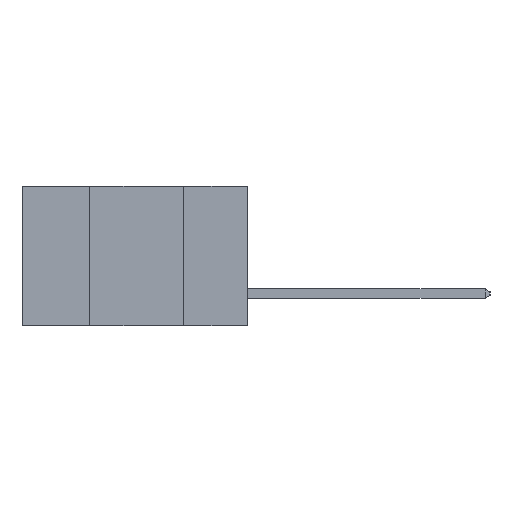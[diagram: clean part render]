
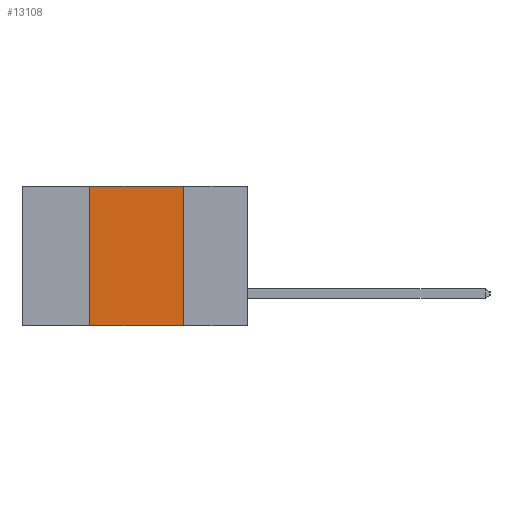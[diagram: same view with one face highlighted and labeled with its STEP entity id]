
A CAD part, left-side view. The second image highlights one B-rep face of the part: STEP entity #13108.
In plain terms, the highlighted planar face has unit normal (-1, 0, 0).
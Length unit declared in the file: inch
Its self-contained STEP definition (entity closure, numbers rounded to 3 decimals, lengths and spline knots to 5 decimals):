
#719 = EDGE_CURVE ( 'NONE', #11733, #8810, #9174, .T. ) ;
#1313 = VECTOR ( 'NONE', #2864, 39.37008 ) ;
#1465 = VECTOR ( 'NONE', #12414, 39.37008 ) ;
#2864 = DIRECTION ( 'NONE',  ( 0., 0., 1. ) ) ;
#2872 = CARTESIAN_POINT ( 'NONE',  ( 0., 0.42, -0.37 ) ) ;
#3395 = ORIENTED_EDGE ( 'NONE', *, *, #7102, .F. ) ;
#3495 = CARTESIAN_POINT ( 'NONE',  ( 0., 0.42, -0.37 ) ) ;
#3544 = ORIENTED_EDGE ( 'NONE', *, *, #719, .T. ) ;
#3562 = AXIS2_PLACEMENT_3D ( 'NONE', #10166, #4051, #11167 ) ;
#3681 = ORIENTED_EDGE ( 'NONE', *, *, #6445, .F. ) ;
#4051 = DIRECTION ( 'NONE',  ( 1., 0., 0. ) ) ;
#4271 = VERTEX_POINT ( 'NONE', #12427 ) ;
#5142 = LINE ( 'NONE', #10914, #7235 ) ;
#6215 = FACE_OUTER_BOUND ( 'NONE', #8141, .T. ) ;
#6445 = EDGE_CURVE ( 'NONE', #4271, #8810, #5142, .T. ) ;
#6952 = ORIENTED_EDGE ( 'NONE', *, *, #10053, .F. ) ;
#7055 = LINE ( 'NONE', #12461, #1465 ) ;
#7065 = CARTESIAN_POINT ( 'NONE',  ( 0., 0.42, 0. ) ) ;
#7102 = EDGE_CURVE ( 'NONE', #9390, #4271, #7055, .T. ) ;
#7235 = VECTOR ( 'NONE', #10649, 39.37008 ) ;
#8141 = EDGE_LOOP ( 'NONE', ( #3681, #3395, #6952, #3544 ) ) ;
#8810 = VERTEX_POINT ( 'NONE', #10860 ) ;
#9174 = LINE ( 'NONE', #11252, #11526 ) ;
#9277 = LINE ( 'NONE', #2872, #1313 ) ;
#9390 = VERTEX_POINT ( 'NONE', #7065 ) ;
#10053 = EDGE_CURVE ( 'NONE', #11733, #9390, #9277, .T. ) ;
#10166 = CARTESIAN_POINT ( 'NONE',  ( 0., 0.6, 0. ) ) ;
#10649 = DIRECTION ( 'NONE',  ( 0., 0., -1. ) ) ;
#10860 = CARTESIAN_POINT ( 'NONE',  ( 0., 0.17, -0.37 ) ) ;
#10914 = CARTESIAN_POINT ( 'NONE',  ( 0., 0.17, -0.37 ) ) ;
#11122 = PLANE ( 'NONE',  #3562 ) ;
#11167 = DIRECTION ( 'NONE',  ( 0., 0., -1. ) ) ;
#11252 = CARTESIAN_POINT ( 'NONE',  ( 0., 0.6, -0.37 ) ) ;
#11526 = VECTOR ( 'NONE', #12684, 39.37008 ) ;
#11733 = VERTEX_POINT ( 'NONE', #3495 ) ;
#12414 = DIRECTION ( 'NONE',  ( 0., -1., 0. ) ) ;
#12427 = CARTESIAN_POINT ( 'NONE',  ( 0., 0.17, 0. ) ) ;
#12461 = CARTESIAN_POINT ( 'NONE',  ( 0., 0.6, 0. ) ) ;
#12684 = DIRECTION ( 'NONE',  ( 0., -1., 0. ) ) ;
#13108 = ADVANCED_FACE ( 'NONE', ( #6215 ), #11122, .F. ) ;
